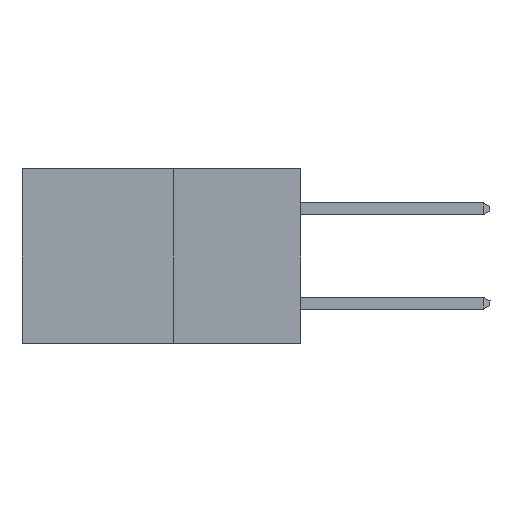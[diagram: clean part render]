
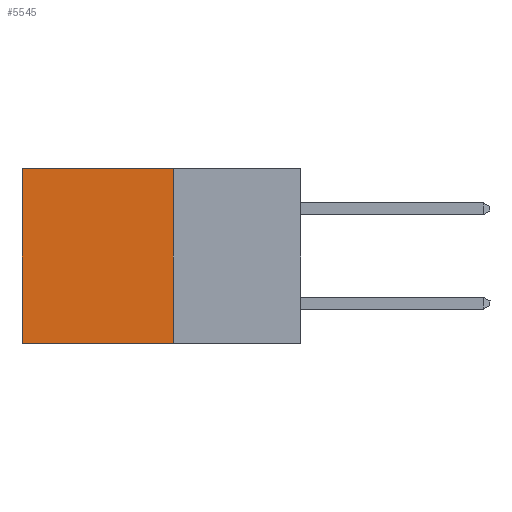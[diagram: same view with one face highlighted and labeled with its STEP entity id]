
A CAD part, left-side view. The second image highlights one B-rep face of the part: STEP entity #5545.
In plain terms, the highlighted planar face has unit normal (-1, 0, 0).
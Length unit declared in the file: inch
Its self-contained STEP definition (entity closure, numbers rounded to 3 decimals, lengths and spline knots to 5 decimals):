
#1 = DIRECTION ( 'NONE',  ( 0., 0., -1. ) ) ;
#356 = CARTESIAN_POINT ( 'NONE',  ( 0.277, 0.27, 0. ) ) ;
#605 = VERTEX_POINT ( 'NONE', #29775 ) ;
#671 = ORIENTED_EDGE ( 'NONE', *, *, #18401, .T. ) ;
#1026 = LINE ( 'NONE', #4496, #20304 ) ;
#1147 = LINE ( 'NONE', #2832, #12841 ) ;
#1711 = DIRECTION ( 'NONE',  ( 0., 1., 0. ) ) ;
#2832 = CARTESIAN_POINT ( 'NONE',  ( 0.277, 0.27, -0.37 ) ) ;
#3438 = DIRECTION ( 'NONE',  ( 0., 0., -1. ) ) ;
#3577 = DIRECTION ( 'NONE',  ( 1., 0., 0. ) ) ;
#4496 = CARTESIAN_POINT ( 'NONE',  ( 0.277, 0.27, -0.37 ) ) ;
#4769 = CARTESIAN_POINT ( 'NONE',  ( 0.277, 0.59, -0.37 ) ) ;
#4913 = ORIENTED_EDGE ( 'NONE', *, *, #26777, .T. ) ;
#5186 = DIRECTION ( 'NONE',  ( 0., 0., -1. ) ) ;
#5545 = ADVANCED_FACE ( 'NONE', ( #11339 ), #5856, .F. ) ;
#5856 = PLANE ( 'NONE',  #28540 ) ;
#6742 = VECTOR ( 'NONE', #1711, 39.37008 ) ;
#10205 = ORIENTED_EDGE ( 'NONE', *, *, #20228, .F. ) ;
#11094 = VERTEX_POINT ( 'NONE', #4769 ) ;
#11179 = CARTESIAN_POINT ( 'NONE',  ( 0.277, 0.59, 0. ) ) ;
#11339 = FACE_OUTER_BOUND ( 'NONE', #29513, .T. ) ;
#12841 = VECTOR ( 'NONE', #5186, 39.37008 ) ;
#15622 = CARTESIAN_POINT ( 'NONE',  ( 0.277, 0.27, 0. ) ) ;
#16907 = ORIENTED_EDGE ( 'NONE', *, *, #26715, .F. ) ;
#17226 = VERTEX_POINT ( 'NONE', #356 ) ;
#18401 = EDGE_CURVE ( 'NONE', #17226, #19163, #25270, .T. ) ;
#19163 = VERTEX_POINT ( 'NONE', #11179 ) ;
#20228 = EDGE_CURVE ( 'NONE', #17226, #605, #1147, .T. ) ;
#20304 = VECTOR ( 'NONE', #22982, 39.37008 ) ;
#20959 = CARTESIAN_POINT ( 'NONE',  ( 0.277, 0.59, -0.37 ) ) ;
#22982 = DIRECTION ( 'NONE',  ( 0., 1., 0. ) ) ;
#24317 = VECTOR ( 'NONE', #1, 39.37008 ) ;
#25270 = LINE ( 'NONE', #15622, #6742 ) ;
#26594 = CARTESIAN_POINT ( 'NONE',  ( 0.277, 0.27, -0.37 ) ) ;
#26715 = EDGE_CURVE ( 'NONE', #605, #11094, #1026, .T. ) ;
#26777 = EDGE_CURVE ( 'NONE', #19163, #11094, #29677, .T. ) ;
#28540 = AXIS2_PLACEMENT_3D ( 'NONE', #26594, #3577, #3438 ) ;
#29513 = EDGE_LOOP ( 'NONE', ( #4913, #16907, #10205, #671 ) ) ;
#29677 = LINE ( 'NONE', #20959, #24317 ) ;
#29775 = CARTESIAN_POINT ( 'NONE',  ( 0.277, 0.27, -0.37 ) ) ;
